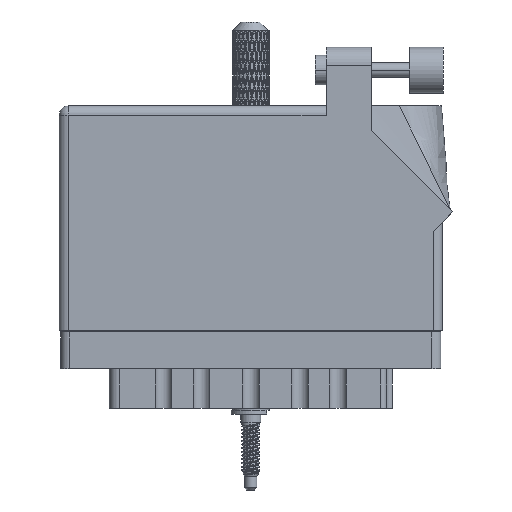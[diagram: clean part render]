
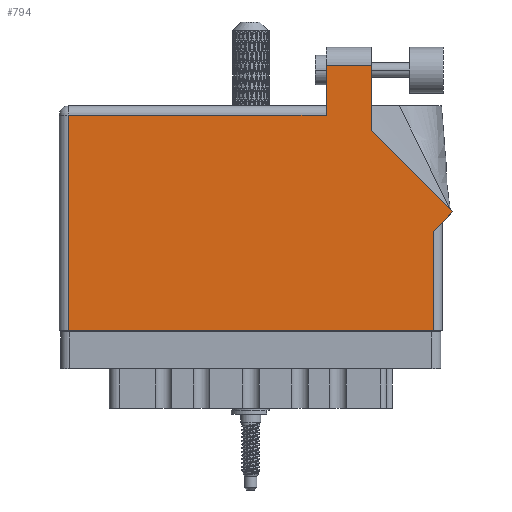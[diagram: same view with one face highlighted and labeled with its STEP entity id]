
A CAD part, front view. The second image highlights one B-rep face of the part: STEP entity #794.
In plain terms, the highlighted face is planar.
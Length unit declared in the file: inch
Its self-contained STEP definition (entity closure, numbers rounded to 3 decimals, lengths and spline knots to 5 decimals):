
#595 = DIRECTION ( 'NONE',  ( 0., -1., 0. ) ) ;
#794 = ADVANCED_FACE ( 'NONE', ( #81620 ), #63686, .F. ) ;
#2344 = DIRECTION ( 'NONE',  ( -1., 0., 0. ) ) ;
#5021 = LINE ( 'NONE', #109495, #105896 ) ;
#5784 = VERTEX_POINT ( 'NONE', #26557 ) ;
#6618 = CARTESIAN_POINT ( 'NONE',  ( 2.612, 0.737, 0. ) ) ;
#8441 = DIRECTION ( 'NONE',  ( -1., 0., 0. ) ) ;
#9037 = EDGE_CURVE ( 'NONE', #47305, #103520, #113021, .T. ) ;
#9568 = ORIENTED_EDGE ( 'NONE', *, *, #49285, .T. ) ;
#10147 = ORIENTED_EDGE ( 'NONE', *, *, #84367, .T. ) ;
#13073 = CARTESIAN_POINT ( 'NONE',  ( 2.55, 0.737, 0. ) ) ;
#13916 = EDGE_LOOP ( 'NONE', ( #71831, #60489, #61893, #10147, #9568, #14967, #48078, #114118, #21857 ) ) ;
#14967 = ORIENTED_EDGE ( 'NONE', *, *, #87962, .T. ) ;
#15778 = VERTEX_POINT ( 'NONE', #111736 ) ;
#18325 = LINE ( 'NONE', #115575, #58569 ) ;
#21519 = VERTEX_POINT ( 'NONE', #90703 ) ;
#21857 = ORIENTED_EDGE ( 'NONE', *, *, #109387, .T. ) ;
#22442 = LINE ( 'NONE', #111458, #98778 ) ;
#23111 = AXIS2_PLACEMENT_3D ( 'NONE', #25517, #90322, #34780 ) ;
#25517 = CARTESIAN_POINT ( 'NONE',  ( 0., 1.53, 0. ) ) ;
#26557 = CARTESIAN_POINT ( 'NONE',  ( 2.68271, 0.80771, 0. ) ) ;
#26605 = CARTESIAN_POINT ( 'NONE',  ( 2.126, 1.805, 0. ) ) ;
#30481 = EDGE_CURVE ( 'NONE', #42488, #84995, #74503, .T. ) ;
#32917 = CARTESIAN_POINT ( 'NONE',  ( 2.68271, 0.80771, 0. ) ) ;
#34780 = DIRECTION ( 'NONE',  ( -1., 0., 0. ) ) ;
#37849 = VECTOR ( 'NONE', #2344, 39.37008 ) ;
#38100 = VECTOR ( 'NONE', #51419, 39.37008 ) ;
#39168 = EDGE_CURVE ( 'NONE', #103520, #42214, #5021, .T. ) ;
#42214 = VERTEX_POINT ( 'NONE', #59458 ) ;
#42488 = VERTEX_POINT ( 'NONE', #93351 ) ;
#47305 = VERTEX_POINT ( 'NONE', #53237 ) ;
#48078 = ORIENTED_EDGE ( 'NONE', *, *, #30481, .T. ) ;
#49285 = EDGE_CURVE ( 'NONE', #21519, #15778, #22442, .T. ) ;
#51419 = DIRECTION ( 'NONE',  ( 0., 1., 0. ) ) ;
#53237 = CARTESIAN_POINT ( 'NONE',  ( 2.126, 1.36442, 0. ) ) ;
#58569 = VECTOR ( 'NONE', #98632, 39.37008 ) ;
#59458 = CARTESIAN_POINT ( 'NONE',  ( 1.819, 1.805, 0. ) ) ;
#60489 = ORIENTED_EDGE ( 'NONE', *, *, #39168, .T. ) ;
#61043 = DIRECTION ( 'NONE',  ( -0.707, 0.707, 0. ) ) ;
#61893 = ORIENTED_EDGE ( 'NONE', *, *, #97080, .T. ) ;
#63686 = PLANE ( 'NONE',  #23111 ) ;
#68017 = LINE ( 'NONE', #104638, #37849 ) ;
#71831 = ORIENTED_EDGE ( 'NONE', *, *, #9037, .T. ) ;
#74503 = LINE ( 'NONE', #13073, #94823 ) ;
#80406 = CARTESIAN_POINT ( 'NONE',  ( 2.126, 1.36442, 0. ) ) ;
#81620 = FACE_OUTER_BOUND ( 'NONE', #13916, .T. ) ;
#84367 = EDGE_CURVE ( 'NONE', #98222, #21519, #68017, .T. ) ;
#84369 = DIRECTION ( 'NONE',  ( 0., -1., 0. ) ) ;
#84995 = VERTEX_POINT ( 'NONE', #99433 ) ;
#87962 = EDGE_CURVE ( 'NONE', #15778, #42488, #18325, .T. ) ;
#89125 = LINE ( 'NONE', #92385, #110683 ) ;
#90322 = DIRECTION ( 'NONE',  ( 0., 0., -1. ) ) ;
#90703 = CARTESIAN_POINT ( 'NONE',  ( 0.062, 1.468, 0. ) ) ;
#92385 = CARTESIAN_POINT ( 'NONE',  ( 1.819, 1.53, 0. ) ) ;
#93351 = CARTESIAN_POINT ( 'NONE',  ( 2.55, 0., 0. ) ) ;
#93986 = CARTESIAN_POINT ( 'NONE',  ( 1.819, 1.468, 0. ) ) ;
#94794 = DIRECTION ( 'NONE',  ( 0., 1., 0. ) ) ;
#94823 = VECTOR ( 'NONE', #94794, 39.37008 ) ;
#96376 = VECTOR ( 'NONE', #107300, 39.37008 ) ;
#97080 = EDGE_CURVE ( 'NONE', #42214, #98222, #89125, .T. ) ;
#98222 = VERTEX_POINT ( 'NONE', #93986 ) ;
#98632 = DIRECTION ( 'NONE',  ( 1., 0., 0. ) ) ;
#98778 = VECTOR ( 'NONE', #84369, 39.37008 ) ;
#99433 = CARTESIAN_POINT ( 'NONE',  ( 2.55, 0.675, 0. ) ) ;
#103520 = VERTEX_POINT ( 'NONE', #26605 ) ;
#104638 = CARTESIAN_POINT ( 'NONE',  ( 0., 1.468, 0. ) ) ;
#105772 = EDGE_CURVE ( 'NONE', #84995, #5784, #110799, .T. ) ;
#105896 = VECTOR ( 'NONE', #8441, 39.37008 ) ;
#107300 = DIRECTION ( 'NONE',  ( 0.707, 0.707, 0. ) ) ;
#109387 = EDGE_CURVE ( 'NONE', #5784, #47305, #119055, .T. ) ;
#109495 = CARTESIAN_POINT ( 'NONE',  ( 1.819, 1.805, 0. ) ) ;
#110683 = VECTOR ( 'NONE', #595, 39.37008 ) ;
#110799 = LINE ( 'NONE', #6618, #96376 ) ;
#111458 = CARTESIAN_POINT ( 'NONE',  ( 0.062, 0., 0. ) ) ;
#111736 = CARTESIAN_POINT ( 'NONE',  ( 0.062, 0., 0. ) ) ;
#113021 = LINE ( 'NONE', #80406, #38100 ) ;
#113303 = VECTOR ( 'NONE', #61043, 39.37008 ) ;
#114118 = ORIENTED_EDGE ( 'NONE', *, *, #105772, .T. ) ;
#115575 = CARTESIAN_POINT ( 'NONE',  ( 0., 0., 0. ) ) ;
#119055 = LINE ( 'NONE', #32917, #113303 ) ;
